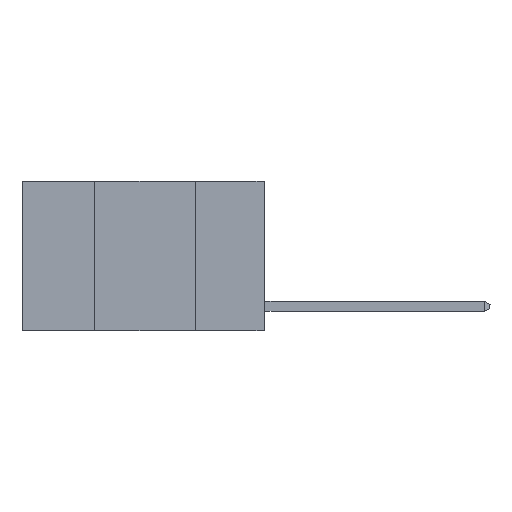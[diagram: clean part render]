
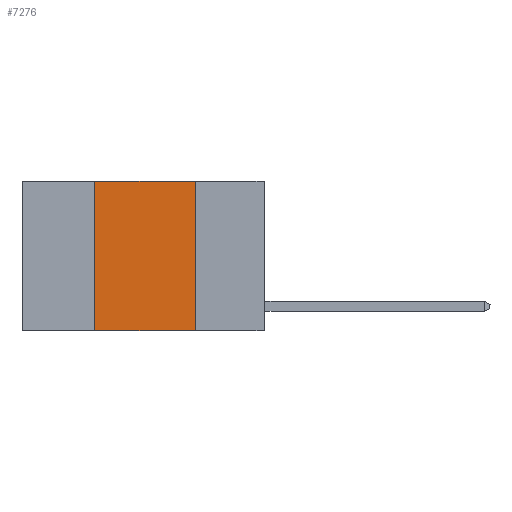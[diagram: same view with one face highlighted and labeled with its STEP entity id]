
A CAD part, left-side view. The second image highlights one B-rep face of the part: STEP entity #7276.
In plain terms, the highlighted planar face has unit normal (-1, 0, 0).
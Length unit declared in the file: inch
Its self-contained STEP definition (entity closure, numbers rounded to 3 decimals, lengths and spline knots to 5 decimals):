
#710 = EDGE_CURVE ( 'NONE', #4586, #1245, #10061, .T. ) ;
#1245 = VERTEX_POINT ( 'NONE', #1473 ) ;
#1473 = CARTESIAN_POINT ( 'NONE',  ( 0., 0.17, 0. ) ) ;
#1984 = LINE ( 'NONE', #13177, #19010 ) ;
#2137 = CARTESIAN_POINT ( 'NONE',  ( 0., 0.6, -0.37 ) ) ;
#2711 = AXIS2_PLACEMENT_3D ( 'NONE', #16690, #16760, #6914 ) ;
#3929 = VERTEX_POINT ( 'NONE', #11359 ) ;
#4151 = ORIENTED_EDGE ( 'NONE', *, *, #20155, .F. ) ;
#4394 = LINE ( 'NONE', #15605, #4912 ) ;
#4586 = VERTEX_POINT ( 'NONE', #18226 ) ;
#4912 = VECTOR ( 'NONE', #17237, 39.37008 ) ;
#4974 = DIRECTION ( 'NONE',  ( 0., 0., 1. ) ) ;
#5168 = VECTOR ( 'NONE', #18593, 39.37008 ) ;
#5260 = PLANE ( 'NONE',  #2711 ) ;
#6225 = ORIENTED_EDGE ( 'NONE', *, *, #7360, .T. ) ;
#6914 = DIRECTION ( 'NONE',  ( 0., 0., -1. ) ) ;
#7276 = ADVANCED_FACE ( 'NONE', ( #9964 ), #5260, .F. ) ;
#7360 = EDGE_CURVE ( 'NONE', #12449, #3929, #17151, .T. ) ;
#8395 = VECTOR ( 'NONE', #15260, 39.37008 ) ;
#9964 = FACE_OUTER_BOUND ( 'NONE', #19448, .T. ) ;
#10061 = LINE ( 'NONE', #18675, #5168 ) ;
#10567 = EDGE_CURVE ( 'NONE', #12449, #4586, #1984, .T. ) ;
#11359 = CARTESIAN_POINT ( 'NONE',  ( 0., 0.17, -0.37 ) ) ;
#12449 = VERTEX_POINT ( 'NONE', #13819 ) ;
#13177 = CARTESIAN_POINT ( 'NONE',  ( 0., 0.42, 0. ) ) ;
#13422 = ORIENTED_EDGE ( 'NONE', *, *, #10567, .F. ) ;
#13819 = CARTESIAN_POINT ( 'NONE',  ( 0., 0.42, -0.37 ) ) ;
#15260 = DIRECTION ( 'NONE',  ( 0., -1., 0. ) ) ;
#15605 = CARTESIAN_POINT ( 'NONE',  ( 0., 0.17, 0. ) ) ;
#16690 = CARTESIAN_POINT ( 'NONE',  ( 0., 0.6, 0. ) ) ;
#16760 = DIRECTION ( 'NONE',  ( 1., 0., 0. ) ) ;
#17151 = LINE ( 'NONE', #2137, #8395 ) ;
#17237 = DIRECTION ( 'NONE',  ( 0., 0., -1. ) ) ;
#17260 = ORIENTED_EDGE ( 'NONE', *, *, #710, .F. ) ;
#18226 = CARTESIAN_POINT ( 'NONE',  ( 0., 0.42, 0. ) ) ;
#18593 = DIRECTION ( 'NONE',  ( 0., -1., 0. ) ) ;
#18675 = CARTESIAN_POINT ( 'NONE',  ( 0., 0.6, 0. ) ) ;
#19010 = VECTOR ( 'NONE', #4974, 39.37008 ) ;
#19448 = EDGE_LOOP ( 'NONE', ( #4151, #17260, #13422, #6225 ) ) ;
#20155 = EDGE_CURVE ( 'NONE', #1245, #3929, #4394, .T. ) ;
